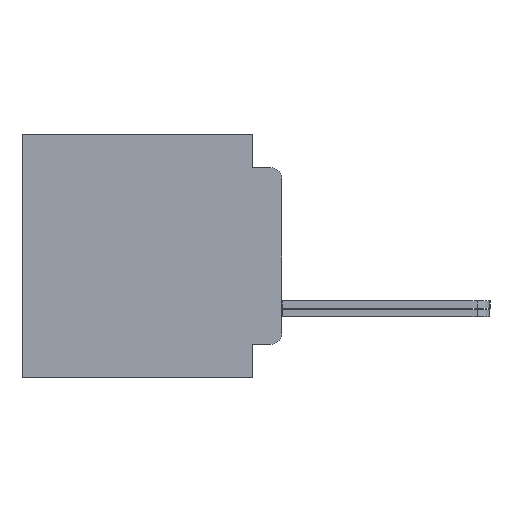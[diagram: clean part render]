
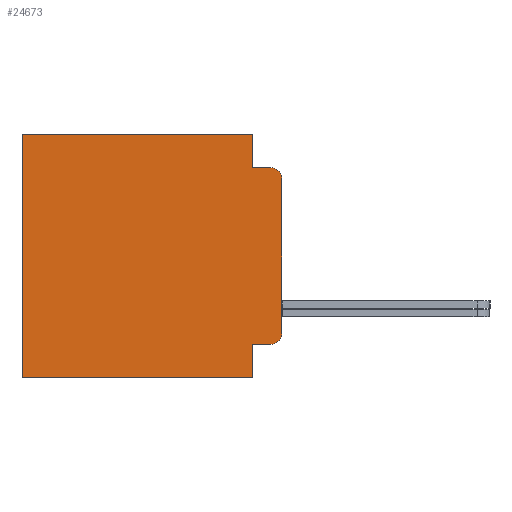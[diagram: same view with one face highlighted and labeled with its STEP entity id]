
A CAD part, left-side view. The second image highlights one B-rep face of the part: STEP entity #24673.
In plain terms, the highlighted planar face has unit normal (-1, 0, 0).
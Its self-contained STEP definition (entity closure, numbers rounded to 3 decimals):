
#97 = DIRECTION ( 'NONE',  ( 0., 0., -1. ) ) ;
#226 = EDGE_CURVE ( 'NONE', #25928, #2811, #10019, .T. ) ;
#945 = EDGE_CURVE ( 'NONE', #3606, #8972, #25223, .T. ) ;
#949 = CARTESIAN_POINT ( 'NONE',  ( -67.462, 1.295, 3.975 ) ) ;
#969 = CARTESIAN_POINT ( 'NONE',  ( -67.462, 0., -5.486 ) ) ;
#1983 = LINE ( 'NONE', #969, #25369 ) ;
#2053 = VERTEX_POINT ( 'NONE', #9038 ) ;
#2090 = CARTESIAN_POINT ( 'NONE',  ( -67.462, 1.295, 3.975 ) ) ;
#2811 = VERTEX_POINT ( 'NONE', #24909 ) ;
#3308 = LINE ( 'NONE', #13755, #25036 ) ;
#3606 = VERTEX_POINT ( 'NONE', #19584 ) ;
#3905 = EDGE_CURVE ( 'NONE', #2053, #14140, #12419, .T. ) ;
#4085 = ORIENTED_EDGE ( 'NONE', *, *, #15477, .T. ) ;
#5469 = VECTOR ( 'NONE', #16723, 1000. ) ;
#5855 = VECTOR ( 'NONE', #18458, 1000. ) ;
#7033 = VERTEX_POINT ( 'NONE', #24387 ) ;
#7100 = CARTESIAN_POINT ( 'NONE',  ( -67.462, 0., 3.467 ) ) ;
#7329 = ORIENTED_EDGE ( 'NONE', *, *, #15744, .F. ) ;
#7471 = EDGE_CURVE ( 'NONE', #2811, #7033, #24099, .T. ) ;
#7607 = EDGE_CURVE ( 'NONE', #9252, #7033, #1983, .T. ) ;
#8531 = EDGE_CURVE ( 'NONE', #17487, #23784, #25046, .T. ) ;
#8652 = CARTESIAN_POINT ( 'NONE',  ( -67.462, 11.684, -5.486 ) ) ;
#8864 = LINE ( 'NONE', #16883, #9530 ) ;
#8938 = EDGE_CURVE ( 'NONE', #25928, #2053, #8864, .T. ) ;
#8972 = VERTEX_POINT ( 'NONE', #27285 ) ;
#9038 = CARTESIAN_POINT ( 'NONE',  ( -67.462, 1.295, -5.486 ) ) ;
#9252 = VERTEX_POINT ( 'NONE', #7100 ) ;
#9343 = AXIS2_PLACEMENT_3D ( 'NONE', #24720, #12187, #14408 ) ;
#9455 = ORIENTED_EDGE ( 'NONE', *, *, #7607, .F. ) ;
#9530 = VECTOR ( 'NONE', #97, 1000. ) ;
#9752 = DIRECTION ( 'NONE',  ( 0., 0., -1. ) ) ;
#9964 = PLANE ( 'NONE',  #9343 ) ;
#9968 = ORIENTED_EDGE ( 'NONE', *, *, #945, .T. ) ;
#10019 = LINE ( 'NONE', #11397, #24151 ) ;
#10224 = VECTOR ( 'NONE', #25114, 1000. ) ;
#10583 = ORIENTED_EDGE ( 'NONE', *, *, #3905, .F. ) ;
#10637 = CARTESIAN_POINT ( 'NONE',  ( -67.462, 1.295, -3.975 ) ) ;
#11085 = FACE_OUTER_BOUND ( 'NONE', #12925, .T. ) ;
#11397 = CARTESIAN_POINT ( 'NONE',  ( -67.462, 1.295, -3.975 ) ) ;
#11448 = ORIENTED_EDGE ( 'NONE', *, *, #8938, .F. ) ;
#11488 = AXIS2_PLACEMENT_3D ( 'NONE', #17794, #15862, #17703 ) ;
#11818 = CARTESIAN_POINT ( 'NONE',  ( -67.462, 0., -5.486 ) ) ;
#11861 = VECTOR ( 'NONE', #21300, 1000. ) ;
#12187 = DIRECTION ( 'NONE',  ( 1., 0., 0. ) ) ;
#12387 = ORIENTED_EDGE ( 'NONE', *, *, #7471, .T. ) ;
#12419 = LINE ( 'NONE', #11818, #5855 ) ;
#12925 = EDGE_LOOP ( 'NONE', ( #26452, #12387, #9455, #24451, #26219, #7329, #9968, #4085, #10583, #11448 ) ) ;
#13203 = LINE ( 'NONE', #8652, #11861 ) ;
#13755 = CARTESIAN_POINT ( 'NONE',  ( -67.462, 1.295, 0. ) ) ;
#14140 = VERTEX_POINT ( 'NONE', #14708 ) ;
#14408 = DIRECTION ( 'NONE',  ( 0., 0., -1. ) ) ;
#14708 = CARTESIAN_POINT ( 'NONE',  ( -67.462, 11.684, -5.486 ) ) ;
#15352 = DIRECTION ( 'NONE',  ( -1., 0., 0. ) ) ;
#15477 = EDGE_CURVE ( 'NONE', #8972, #14140, #13203, .T. ) ;
#15744 = EDGE_CURVE ( 'NONE', #3606, #17487, #3308, .T. ) ;
#15862 = DIRECTION ( 'NONE',  ( -1., 0., 0. ) ) ;
#15887 = DIRECTION ( 'NONE',  ( 0., 0., -1. ) ) ;
#16723 = DIRECTION ( 'NONE',  ( 0., 1., 0. ) ) ;
#16883 = CARTESIAN_POINT ( 'NONE',  ( -67.462, 1.295, 0. ) ) ;
#17436 = EDGE_CURVE ( 'NONE', #9252, #23784, #26967, .T. ) ;
#17487 = VERTEX_POINT ( 'NONE', #949 ) ;
#17640 = DIRECTION ( 'NONE',  ( 0., 0., -1. ) ) ;
#17703 = DIRECTION ( 'NONE',  ( 0., 0., -1. ) ) ;
#17794 = CARTESIAN_POINT ( 'NONE',  ( -67.462, 0.508, 3.467 ) ) ;
#18458 = DIRECTION ( 'NONE',  ( 0., 1., 0. ) ) ;
#19584 = CARTESIAN_POINT ( 'NONE',  ( -67.462, 1.295, 5.486 ) ) ;
#19676 = CARTESIAN_POINT ( 'NONE',  ( -67.462, 0.508, -3.467 ) ) ;
#21142 = CARTESIAN_POINT ( 'NONE',  ( -67.462, 0., 5.486 ) ) ;
#21300 = DIRECTION ( 'NONE',  ( 0., 0., -1. ) ) ;
#23784 = VERTEX_POINT ( 'NONE', #24122 ) ;
#23941 = DIRECTION ( 'NONE',  ( 0., -1., 0. ) ) ;
#24099 = CIRCLE ( 'NONE', #25956, 0.508 ) ;
#24122 = CARTESIAN_POINT ( 'NONE',  ( -67.462, 0.508, 3.975 ) ) ;
#24151 = VECTOR ( 'NONE', #23941, 1000. ) ;
#24387 = CARTESIAN_POINT ( 'NONE',  ( -67.462, 0., -3.467 ) ) ;
#24451 = ORIENTED_EDGE ( 'NONE', *, *, #17436, .T. ) ;
#24673 = ADVANCED_FACE ( 'NONE', ( #11085 ), #9964, .F. ) ;
#24720 = CARTESIAN_POINT ( 'NONE',  ( -67.462, 0., -5.486 ) ) ;
#24909 = CARTESIAN_POINT ( 'NONE',  ( -67.462, 0.508, -3.975 ) ) ;
#25036 = VECTOR ( 'NONE', #9752, 1000. ) ;
#25046 = LINE ( 'NONE', #2090, #10224 ) ;
#25114 = DIRECTION ( 'NONE',  ( 0., -1., 0. ) ) ;
#25223 = LINE ( 'NONE', #21142, #5469 ) ;
#25369 = VECTOR ( 'NONE', #15887, 1000. ) ;
#25928 = VERTEX_POINT ( 'NONE', #10637 ) ;
#25956 = AXIS2_PLACEMENT_3D ( 'NONE', #19676, #15352, #17640 ) ;
#26219 = ORIENTED_EDGE ( 'NONE', *, *, #8531, .F. ) ;
#26452 = ORIENTED_EDGE ( 'NONE', *, *, #226, .T. ) ;
#26967 = CIRCLE ( 'NONE', #11488, 0.508 ) ;
#27285 = CARTESIAN_POINT ( 'NONE',  ( -67.462, 11.684, 5.486 ) ) ;
